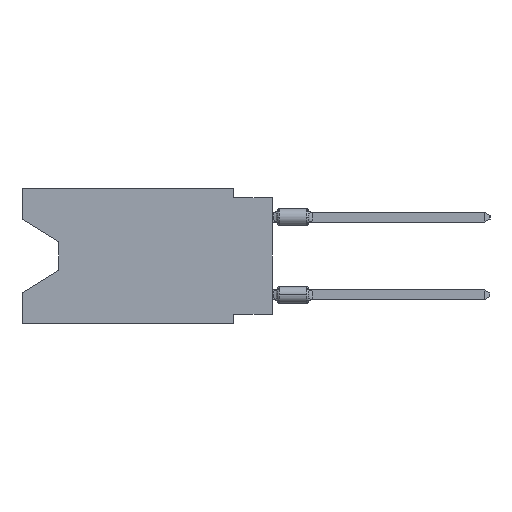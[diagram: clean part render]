
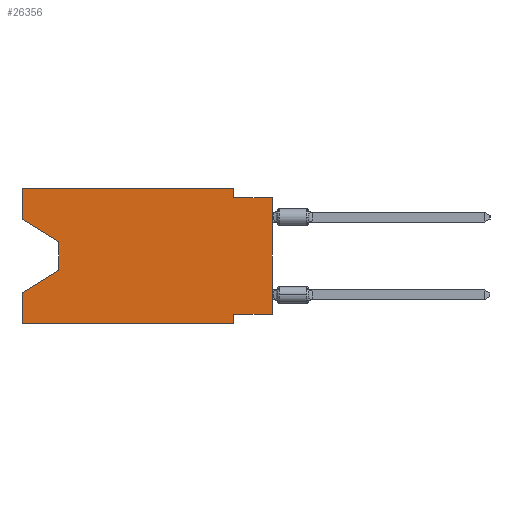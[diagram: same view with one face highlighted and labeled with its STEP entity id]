
A CAD part, left-side view. The second image highlights one B-rep face of the part: STEP entity #26356.
In plain terms, the highlighted planar face has unit normal (-1, 0, 0).
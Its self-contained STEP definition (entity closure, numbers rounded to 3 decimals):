
#835 = ORIENTED_EDGE ( 'NONE', *, *, #21639, .T. ) ;
#1260 = CARTESIAN_POINT ( 'NONE',  ( 0., 2.54, -0.635 ) ) ;
#1552 = VECTOR ( 'NONE', #12156, 1000. ) ;
#1903 = EDGE_CURVE ( 'NONE', #47803, #53422, #23474, .T. ) ;
#2023 = CARTESIAN_POINT ( 'NONE',  ( 0., 16.383, -8.89 ) ) ;
#3019 = DIRECTION ( 'NONE',  ( 0., 0., 1. ) ) ;
#3412 = CARTESIAN_POINT ( 'NONE',  ( 0., 0., -8.255 ) ) ;
#3871 = CARTESIAN_POINT ( 'NONE',  ( 0., 0., -0.635 ) ) ;
#4859 = DIRECTION ( 'NONE',  ( 0., 0.855, -0.519 ) ) ;
#5690 = VECTOR ( 'NONE', #3019, 1000. ) ;
#5814 = CARTESIAN_POINT ( 'NONE',  ( 0., 16.383, -2.038 ) ) ;
#6867 = EDGE_CURVE ( 'NONE', #62379, #45954, #48570, .T. ) ;
#7693 = EDGE_CURVE ( 'NONE', #53422, #39558, #29838, .T. ) ;
#7723 = VECTOR ( 'NONE', #38163, 1000. ) ;
#7912 = CARTESIAN_POINT ( 'NONE',  ( 0., 16.383, 0. ) ) ;
#8594 = DIRECTION ( 'NONE',  ( 0., 1., 0. ) ) ;
#9168 = CARTESIAN_POINT ( 'NONE',  ( 0., 16.383, 0. ) ) ;
#9816 = LINE ( 'NONE', #49413, #27213 ) ;
#11007 = VECTOR ( 'NONE', #4859, 1000. ) ;
#12156 = DIRECTION ( 'NONE',  ( 0., -1., 0. ) ) ;
#12219 = VERTEX_POINT ( 'NONE', #22082 ) ;
#12783 = CARTESIAN_POINT ( 'NONE',  ( 0., 16.383, 0. ) ) ;
#13550 = CARTESIAN_POINT ( 'NONE',  ( 0., 2.54, -8.89 ) ) ;
#15203 = CARTESIAN_POINT ( 'NONE',  ( 0., 16.383, 0. ) ) ;
#15879 = VECTOR ( 'NONE', #20400, 1000. ) ;
#16602 = VECTOR ( 'NONE', #63474, 1000. ) ;
#16758 = EDGE_CURVE ( 'NONE', #45954, #55508, #56629, .T. ) ;
#17762 = CARTESIAN_POINT ( 'NONE',  ( 0., 2.54, -8.89 ) ) ;
#19130 = DIRECTION ( 'NONE',  ( 0., -1., 0. ) ) ;
#20134 = VERTEX_POINT ( 'NONE', #1260 ) ;
#20400 = DIRECTION ( 'NONE',  ( 0., 0., 1. ) ) ;
#20685 = DIRECTION ( 'NONE',  ( 0., 0., -1. ) ) ;
#20945 = ORIENTED_EDGE ( 'NONE', *, *, #6867, .F. ) ;
#21152 = VECTOR ( 'NONE', #42752, 1000. ) ;
#21639 = EDGE_CURVE ( 'NONE', #12219, #59952, #36430, .T. ) ;
#22082 = CARTESIAN_POINT ( 'NONE',  ( 0., 16.383, -8.89 ) ) ;
#23355 = CARTESIAN_POINT ( 'NONE',  ( 0., 0., -8.255 ) ) ;
#23474 = LINE ( 'NONE', #43255, #25027 ) ;
#23961 = EDGE_LOOP ( 'NONE', ( #48620, #41573, #57068, #34408, #835, #49072, #34043, #38946, #60405, #37198, #58815, #20945 ) ) ;
#25027 = VECTOR ( 'NONE', #63067, 1000. ) ;
#26356 = ADVANCED_FACE ( 'NONE', ( #54471 ), #50558, .F. ) ;
#27213 = VECTOR ( 'NONE', #48749, 1000. ) ;
#27673 = CARTESIAN_POINT ( 'NONE',  ( 0., 13.97, -3.505 ) ) ;
#28004 = LINE ( 'NONE', #12783, #5690 ) ;
#29086 = AXIS2_PLACEMENT_3D ( 'NONE', #15203, #59982, #20685 ) ;
#29376 = LINE ( 'NONE', #29691, #16602 ) ;
#29691 = CARTESIAN_POINT ( 'NONE',  ( 0., 2.54, 0. ) ) ;
#29838 = LINE ( 'NONE', #63279, #11007 ) ;
#34043 = ORIENTED_EDGE ( 'NONE', *, *, #47523, .F. ) ;
#34276 = CARTESIAN_POINT ( 'NONE',  ( 0., 16.383, 0. ) ) ;
#34408 = ORIENTED_EDGE ( 'NONE', *, *, #53667, .F. ) ;
#35644 = LINE ( 'NONE', #49941, #15879 ) ;
#36430 = LINE ( 'NONE', #2023, #40342 ) ;
#36802 = CARTESIAN_POINT ( 'NONE',  ( 0., 2.54, -8.255 ) ) ;
#36874 = VERTEX_POINT ( 'NONE', #36802 ) ;
#37198 = ORIENTED_EDGE ( 'NONE', *, *, #48755, .F. ) ;
#38163 = DIRECTION ( 'NONE',  ( 0., 0., 1. ) ) ;
#38946 = ORIENTED_EDGE ( 'NONE', *, *, #41241, .T. ) ;
#38985 = CARTESIAN_POINT ( 'NONE',  ( 0., 2.54, 0. ) ) ;
#39558 = VERTEX_POINT ( 'NONE', #63005 ) ;
#40342 = VECTOR ( 'NONE', #60805, 1000. ) ;
#40518 = VECTOR ( 'NONE', #19130, 1000. ) ;
#41241 = EDGE_CURVE ( 'NONE', #62281, #54923, #35644, .T. ) ;
#41573 = ORIENTED_EDGE ( 'NONE', *, *, #1903, .T. ) ;
#41660 = VECTOR ( 'NONE', #8594, 1000. ) ;
#42752 = DIRECTION ( 'NONE',  ( 0., 0., -1. ) ) ;
#43255 = CARTESIAN_POINT ( 'NONE',  ( 0., 13.97, -3.505 ) ) ;
#43434 = LINE ( 'NONE', #3871, #40518 ) ;
#43631 = LINE ( 'NONE', #3412, #41660 ) ;
#45954 = VERTEX_POINT ( 'NONE', #9168 ) ;
#47523 = EDGE_CURVE ( 'NONE', #62281, #36874, #43631, .T. ) ;
#47803 = VERTEX_POINT ( 'NONE', #27673 ) ;
#48570 = LINE ( 'NONE', #34276, #7723 ) ;
#48620 = ORIENTED_EDGE ( 'NONE', *, *, #62091, .T. ) ;
#48749 = DIRECTION ( 'NONE',  ( 0., -0.855, -0.519 ) ) ;
#48755 = EDGE_CURVE ( 'NONE', #55508, #20134, #29376, .T. ) ;
#49072 = ORIENTED_EDGE ( 'NONE', *, *, #63880, .F. ) ;
#49413 = CARTESIAN_POINT ( 'NONE',  ( 0., 16.383, -2.038 ) ) ;
#49941 = CARTESIAN_POINT ( 'NONE',  ( 0., 0., 0. ) ) ;
#50558 = PLANE ( 'NONE',  #29086 ) ;
#53032 = CARTESIAN_POINT ( 'NONE',  ( 0., 0., -0.635 ) ) ;
#53422 = VERTEX_POINT ( 'NONE', #57949 ) ;
#53667 = EDGE_CURVE ( 'NONE', #12219, #39558, #28004, .T. ) ;
#53767 = LINE ( 'NONE', #13550, #21152 ) ;
#54471 = FACE_OUTER_BOUND ( 'NONE', #23961, .T. ) ;
#54923 = VERTEX_POINT ( 'NONE', #53032 ) ;
#55508 = VERTEX_POINT ( 'NONE', #38985 ) ;
#56629 = LINE ( 'NONE', #7912, #1552 ) ;
#57068 = ORIENTED_EDGE ( 'NONE', *, *, #7693, .T. ) ;
#57949 = CARTESIAN_POINT ( 'NONE',  ( 0., 13.97, -5.385 ) ) ;
#58321 = EDGE_CURVE ( 'NONE', #20134, #54923, #43434, .T. ) ;
#58815 = ORIENTED_EDGE ( 'NONE', *, *, #16758, .F. ) ;
#59952 = VERTEX_POINT ( 'NONE', #17762 ) ;
#59982 = DIRECTION ( 'NONE',  ( 1., 0., 0. ) ) ;
#60405 = ORIENTED_EDGE ( 'NONE', *, *, #58321, .F. ) ;
#60805 = DIRECTION ( 'NONE',  ( 0., -1., 0. ) ) ;
#62091 = EDGE_CURVE ( 'NONE', #62379, #47803, #9816, .T. ) ;
#62281 = VERTEX_POINT ( 'NONE', #23355 ) ;
#62379 = VERTEX_POINT ( 'NONE', #5814 ) ;
#63005 = CARTESIAN_POINT ( 'NONE',  ( 0., 16.383, -6.852 ) ) ;
#63067 = DIRECTION ( 'NONE',  ( 0., 0., -1. ) ) ;
#63279 = CARTESIAN_POINT ( 'NONE',  ( 0., 13.97, -5.385 ) ) ;
#63474 = DIRECTION ( 'NONE',  ( 0., 0., -1. ) ) ;
#63880 = EDGE_CURVE ( 'NONE', #36874, #59952, #53767, .T. ) ;
